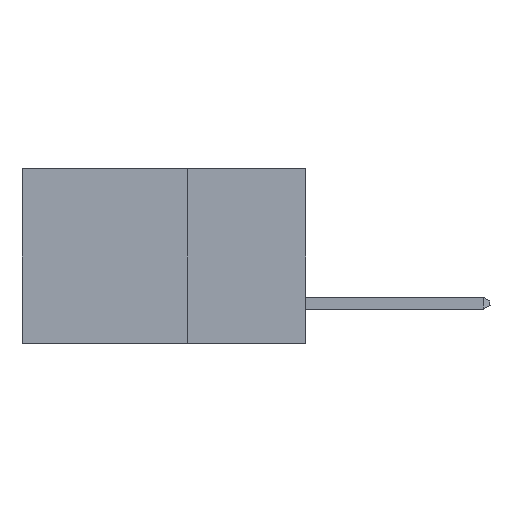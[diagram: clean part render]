
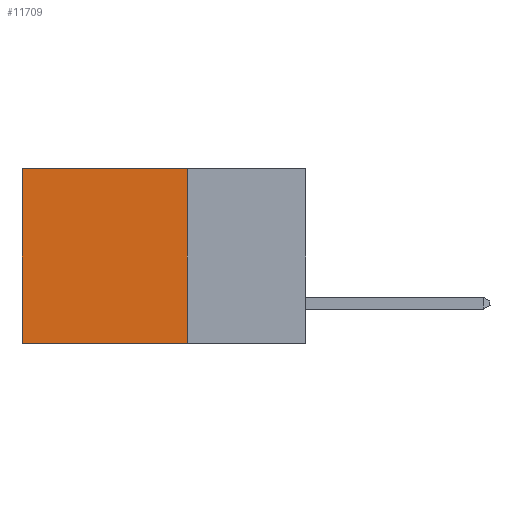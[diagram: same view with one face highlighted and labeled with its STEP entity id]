
A CAD part, left-side view. The second image highlights one B-rep face of the part: STEP entity #11709.
In plain terms, the highlighted planar face has unit normal (-1, 0, 0).
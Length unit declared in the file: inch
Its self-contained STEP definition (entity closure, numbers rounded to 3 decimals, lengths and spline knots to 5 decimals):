
#363 = LINE ( 'NONE', #5115, #13375 ) ;
#1143 = EDGE_CURVE ( 'NONE', #1376, #11137, #2050, .T. ) ;
#1376 = VERTEX_POINT ( 'NONE', #2652 ) ;
#1736 = VERTEX_POINT ( 'NONE', #12342 ) ;
#1773 = CARTESIAN_POINT ( 'NONE',  ( 0.2615, 0.25, -0.37 ) ) ;
#2050 = LINE ( 'NONE', #5514, #4364 ) ;
#2353 = LINE ( 'NONE', #7956, #6973 ) ;
#2540 = EDGE_CURVE ( 'NONE', #1736, #3741, #363, .T. ) ;
#2652 = CARTESIAN_POINT ( 'NONE',  ( 0.2615, 0.25, 0. ) ) ;
#2866 = FACE_OUTER_BOUND ( 'NONE', #3366, .T. ) ;
#3277 = DIRECTION ( 'NONE',  ( 0., 0., -1. ) ) ;
#3287 = CARTESIAN_POINT ( 'NONE',  ( 0.2615, 0.25, 0. ) ) ;
#3366 = EDGE_LOOP ( 'NONE', ( #11167, #5088, #5863, #11811 ) ) ;
#3741 = VERTEX_POINT ( 'NONE', #5910 ) ;
#3823 = DIRECTION ( 'NONE',  ( 1., 0., 0. ) ) ;
#4364 = VECTOR ( 'NONE', #6620, 39.37008 ) ;
#5088 = ORIENTED_EDGE ( 'NONE', *, *, #12406, .F. ) ;
#5115 = CARTESIAN_POINT ( 'NONE',  ( 0.2615, 0.6, -0.37 ) ) ;
#5291 = VECTOR ( 'NONE', #8557, 39.37008 ) ;
#5514 = CARTESIAN_POINT ( 'NONE',  ( 0.2615, 0.25, -0.37 ) ) ;
#5863 = ORIENTED_EDGE ( 'NONE', *, *, #1143, .F. ) ;
#5910 = CARTESIAN_POINT ( 'NONE',  ( 0.2615, 0.6, -0.37 ) ) ;
#6287 = LINE ( 'NONE', #3287, #5291 ) ;
#6620 = DIRECTION ( 'NONE',  ( 0., 0., -1. ) ) ;
#6973 = VECTOR ( 'NONE', #9029, 39.37008 ) ;
#7006 = DIRECTION ( 'NONE',  ( 0., 0., -1. ) ) ;
#7956 = CARTESIAN_POINT ( 'NONE',  ( 0.2615, 0.25, -0.37 ) ) ;
#8276 = CARTESIAN_POINT ( 'NONE',  ( 0.2615, 0.25, -0.37 ) ) ;
#8423 = AXIS2_PLACEMENT_3D ( 'NONE', #1773, #3823, #7006 ) ;
#8557 = DIRECTION ( 'NONE',  ( 0., 1., 0. ) ) ;
#9029 = DIRECTION ( 'NONE',  ( 0., 1., 0. ) ) ;
#10119 = PLANE ( 'NONE',  #8423 ) ;
#11137 = VERTEX_POINT ( 'NONE', #8276 ) ;
#11167 = ORIENTED_EDGE ( 'NONE', *, *, #2540, .T. ) ;
#11709 = ADVANCED_FACE ( 'NONE', ( #2866 ), #10119, .F. ) ;
#11811 = ORIENTED_EDGE ( 'NONE', *, *, #13185, .T. ) ;
#12342 = CARTESIAN_POINT ( 'NONE',  ( 0.2615, 0.6, 0. ) ) ;
#12406 = EDGE_CURVE ( 'NONE', #11137, #3741, #2353, .T. ) ;
#13185 = EDGE_CURVE ( 'NONE', #1376, #1736, #6287, .T. ) ;
#13375 = VECTOR ( 'NONE', #3277, 39.37008 ) ;
